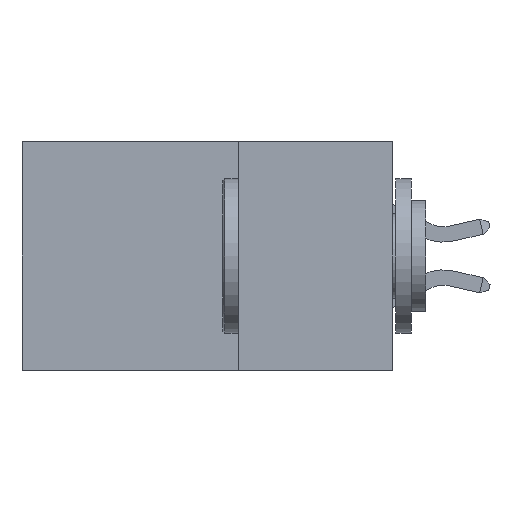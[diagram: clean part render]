
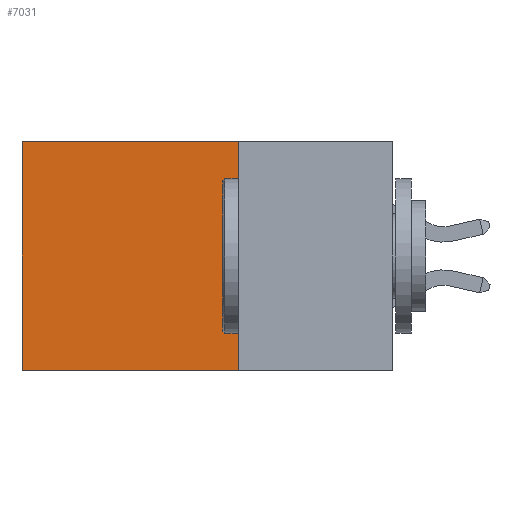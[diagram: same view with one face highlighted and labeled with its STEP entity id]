
A CAD part, left-side view. The second image highlights one B-rep face of the part: STEP entity #7031.
In plain terms, the highlighted planar face has unit normal (-1, 0, 0).
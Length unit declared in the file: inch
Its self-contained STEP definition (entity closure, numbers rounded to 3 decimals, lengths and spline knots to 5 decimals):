
#166 = EDGE_CURVE ( 'NONE', #6334, #3796, #2734, .T. ) ;
#1528 = PLANE ( 'NONE',  #5164 ) ;
#1569 = VECTOR ( 'NONE', #6588, 39.37008 ) ;
#1881 = CARTESIAN_POINT ( 'NONE',  ( 0.2875, 0.6, 0. ) ) ;
#2154 = FACE_OUTER_BOUND ( 'NONE', #4039, .T. ) ;
#2352 = CARTESIAN_POINT ( 'NONE',  ( 0.2875, 0.25, 0. ) ) ;
#2560 = DIRECTION ( 'NONE',  ( 1., 0., 0. ) ) ;
#2648 = LINE ( 'NONE', #4194, #4905 ) ;
#2734 = LINE ( 'NONE', #3572, #6707 ) ;
#2810 = LINE ( 'NONE', #2352, #3242 ) ;
#3242 = VECTOR ( 'NONE', #11544, 39.37008 ) ;
#3367 = CARTESIAN_POINT ( 'NONE',  ( 0.2875, 0.25, 0. ) ) ;
#3572 = CARTESIAN_POINT ( 'NONE',  ( 0.2875, 0.25, 0. ) ) ;
#3796 = VERTEX_POINT ( 'NONE', #1881 ) ;
#4039 = EDGE_LOOP ( 'NONE', ( #6310, #4897, #8920, #5665 ) ) ;
#4194 = CARTESIAN_POINT ( 'NONE',  ( 0.2875, 0.25, -0.37 ) ) ;
#4883 = CARTESIAN_POINT ( 'NONE',  ( 0.2875, 0.6, -0.37 ) ) ;
#4897 = ORIENTED_EDGE ( 'NONE', *, *, #6767, .F. ) ;
#4905 = VECTOR ( 'NONE', #4980, 39.37008 ) ;
#4980 = DIRECTION ( 'NONE',  ( 0., 1., 0. ) ) ;
#5164 = AXIS2_PLACEMENT_3D ( 'NONE', #9710, #2560, #10631 ) ;
#5665 = ORIENTED_EDGE ( 'NONE', *, *, #166, .T. ) ;
#6310 = ORIENTED_EDGE ( 'NONE', *, *, #8100, .T. ) ;
#6334 = VERTEX_POINT ( 'NONE', #3367 ) ;
#6588 = DIRECTION ( 'NONE',  ( 0., 0., -1. ) ) ;
#6707 = VECTOR ( 'NONE', #7966, 39.37008 ) ;
#6767 = EDGE_CURVE ( 'NONE', #9650, #8853, #2648, .T. ) ;
#7031 = ADVANCED_FACE ( 'NONE', ( #2154 ), #1528, .F. ) ;
#7496 = CARTESIAN_POINT ( 'NONE',  ( 0.2875, 0.6, 0. ) ) ;
#7749 = CARTESIAN_POINT ( 'NONE',  ( 0.2875, 0.25, -0.37 ) ) ;
#7966 = DIRECTION ( 'NONE',  ( 0., 1., 0. ) ) ;
#8100 = EDGE_CURVE ( 'NONE', #3796, #8853, #11669, .T. ) ;
#8853 = VERTEX_POINT ( 'NONE', #4883 ) ;
#8920 = ORIENTED_EDGE ( 'NONE', *, *, #9279, .F. ) ;
#9279 = EDGE_CURVE ( 'NONE', #6334, #9650, #2810, .T. ) ;
#9650 = VERTEX_POINT ( 'NONE', #7749 ) ;
#9710 = CARTESIAN_POINT ( 'NONE',  ( 0.2875, 0.25, 0. ) ) ;
#10631 = DIRECTION ( 'NONE',  ( 0., 0., -1. ) ) ;
#11544 = DIRECTION ( 'NONE',  ( 0., 0., -1. ) ) ;
#11669 = LINE ( 'NONE', #7496, #1569 ) ;
